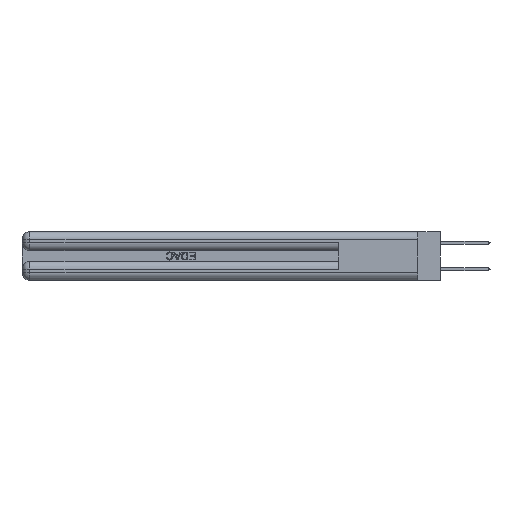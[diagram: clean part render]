
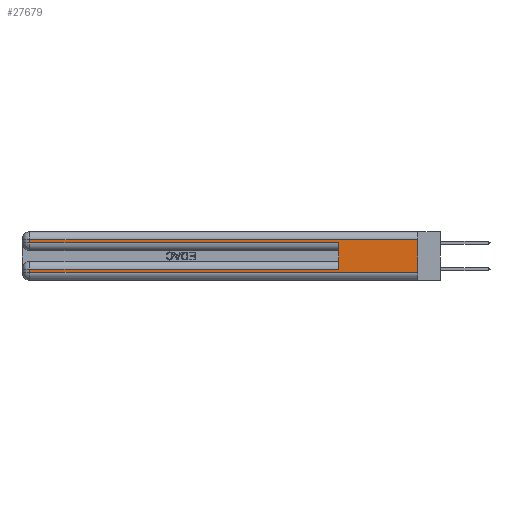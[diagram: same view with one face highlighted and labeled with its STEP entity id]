
A CAD part, left-side view. The second image highlights one B-rep face of the part: STEP entity #27679.
In plain terms, the highlighted planar face has unit normal (-1, 0, 0).
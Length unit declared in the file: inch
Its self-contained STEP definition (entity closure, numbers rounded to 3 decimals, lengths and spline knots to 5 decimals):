
#637 = ORIENTED_EDGE ( 'NONE', *, *, #18047, .T. ) ;
#2802 = EDGE_CURVE ( 'NONE', #39385, #4583, #49757, .T. ) ;
#3992 = VECTOR ( 'NONE', #33472, 39.37008 ) ;
#4583 = VERTEX_POINT ( 'NONE', #31790 ) ;
#5126 = CARTESIAN_POINT ( 'NONE',  ( 0., 0.6, 0.085 ) ) ;
#6220 = DIRECTION ( 'NONE',  ( 0., 0., -1. ) ) ;
#8430 = DIRECTION ( 'NONE',  ( 0., 0., -1. ) ) ;
#10639 = ORIENTED_EDGE ( 'NONE', *, *, #34184, .T. ) ;
#11163 = CARTESIAN_POINT ( 'NONE',  ( 0., 2.94, 0.085 ) ) ;
#11471 = VERTEX_POINT ( 'NONE', #32203 ) ;
#12123 = LINE ( 'NONE', #21710, #22616 ) ;
#14483 = LINE ( 'NONE', #41048, #3992 ) ;
#15492 = CARTESIAN_POINT ( 'NONE',  ( 0., 0., 0.085 ) ) ;
#15514 = DIRECTION ( 'NONE',  ( 0., 0., 1. ) ) ;
#16195 = CARTESIAN_POINT ( 'NONE',  ( 0., 0., 0.37 ) ) ;
#17973 = VERTEX_POINT ( 'NONE', #25187 ) ;
#18047 = EDGE_CURVE ( 'NONE', #4583, #23584, #12123, .T. ) ;
#18401 = ORIENTED_EDGE ( 'NONE', *, *, #41748, .T. ) ;
#20203 = VERTEX_POINT ( 'NONE', #27717 ) ;
#20548 = DIRECTION ( 'NONE',  ( 0., 0., -1. ) ) ;
#21710 = CARTESIAN_POINT ( 'NONE',  ( 0., 0., 0.06 ) ) ;
#22616 = VECTOR ( 'NONE', #25690, 39.37008 ) ;
#22716 = ORIENTED_EDGE ( 'NONE', *, *, #50418, .T. ) ;
#23218 = CARTESIAN_POINT ( 'NONE',  ( 0., 0.6, 0.285 ) ) ;
#23450 = CARTESIAN_POINT ( 'NONE',  ( 0., 0.6, 0.145 ) ) ;
#23584 = VERTEX_POINT ( 'NONE', #46716 ) ;
#25187 = CARTESIAN_POINT ( 'NONE',  ( 0., 2.94, 0.285 ) ) ;
#25690 = DIRECTION ( 'NONE',  ( 0., -1., 0. ) ) ;
#25888 = CARTESIAN_POINT ( 'NONE',  ( 0., 0., 0.37 ) ) ;
#26650 = EDGE_LOOP ( 'NONE', ( #46520, #18401, #10639, #22716, #48410, #44875, #30229, #637 ) ) ;
#26946 = LINE ( 'NONE', #25888, #39701 ) ;
#27377 = DIRECTION ( 'NONE',  ( 0., 1., 0. ) ) ;
#27679 = ADVANCED_FACE ( 'NONE', ( #44504 ), #28084, .F. ) ;
#27717 = CARTESIAN_POINT ( 'NONE',  ( 0., 2.94, 0.31 ) ) ;
#27815 = CARTESIAN_POINT ( 'NONE',  ( 0., 2.94, 0.37 ) ) ;
#28084 = PLANE ( 'NONE',  #49397 ) ;
#29402 = EDGE_CURVE ( 'NONE', #48430, #30035, #47935, .T. ) ;
#29728 = DIRECTION ( 'NONE',  ( 0., -1., 0. ) ) ;
#29775 = VECTOR ( 'NONE', #15514, 39.37008 ) ;
#30035 = VERTEX_POINT ( 'NONE', #23218 ) ;
#30229 = ORIENTED_EDGE ( 'NONE', *, *, #2802, .T. ) ;
#31790 = CARTESIAN_POINT ( 'NONE',  ( 0., 2.94, 0.06 ) ) ;
#32019 = DIRECTION ( 'NONE',  ( 1., 0., 0. ) ) ;
#32203 = CARTESIAN_POINT ( 'NONE',  ( 0., 0., 0.31 ) ) ;
#33472 = DIRECTION ( 'NONE',  ( 0., 1., 0. ) ) ;
#33628 = VECTOR ( 'NONE', #20548, 39.37008 ) ;
#34184 = EDGE_CURVE ( 'NONE', #20203, #17973, #45074, .T. ) ;
#34813 = VECTOR ( 'NONE', #27377, 39.37008 ) ;
#39385 = VERTEX_POINT ( 'NONE', #11163 ) ;
#39503 = VECTOR ( 'NONE', #47269, 39.37008 ) ;
#39701 = VECTOR ( 'NONE', #6220, 39.37008 ) ;
#39998 = CARTESIAN_POINT ( 'NONE',  ( 0., 2.94, 0.37 ) ) ;
#40249 = LINE ( 'NONE', #49023, #44440 ) ;
#40827 = EDGE_CURVE ( 'NONE', #48430, #39385, #45029, .T. ) ;
#41048 = CARTESIAN_POINT ( 'NONE',  ( 0., 0., 0.31 ) ) ;
#41748 = EDGE_CURVE ( 'NONE', #11471, #20203, #14483, .T. ) ;
#44440 = VECTOR ( 'NONE', #29728, 39.37008 ) ;
#44504 = FACE_OUTER_BOUND ( 'NONE', #26650, .T. ) ;
#44875 = ORIENTED_EDGE ( 'NONE', *, *, #40827, .T. ) ;
#45029 = LINE ( 'NONE', #15492, #34813 ) ;
#45074 = LINE ( 'NONE', #39998, #33628 ) ;
#46520 = ORIENTED_EDGE ( 'NONE', *, *, #49710, .F. ) ;
#46716 = CARTESIAN_POINT ( 'NONE',  ( 0., 0., 0.06 ) ) ;
#47269 = DIRECTION ( 'NONE',  ( 0., 0., -1. ) ) ;
#47935 = LINE ( 'NONE', #23450, #29775 ) ;
#48410 = ORIENTED_EDGE ( 'NONE', *, *, #29402, .F. ) ;
#48430 = VERTEX_POINT ( 'NONE', #5126 ) ;
#49023 = CARTESIAN_POINT ( 'NONE',  ( 0., 0., 0.285 ) ) ;
#49397 = AXIS2_PLACEMENT_3D ( 'NONE', #16195, #32019, #8430 ) ;
#49710 = EDGE_CURVE ( 'NONE', #11471, #23584, #26946, .T. ) ;
#49757 = LINE ( 'NONE', #27815, #39503 ) ;
#50418 = EDGE_CURVE ( 'NONE', #17973, #30035, #40249, .T. ) ;
